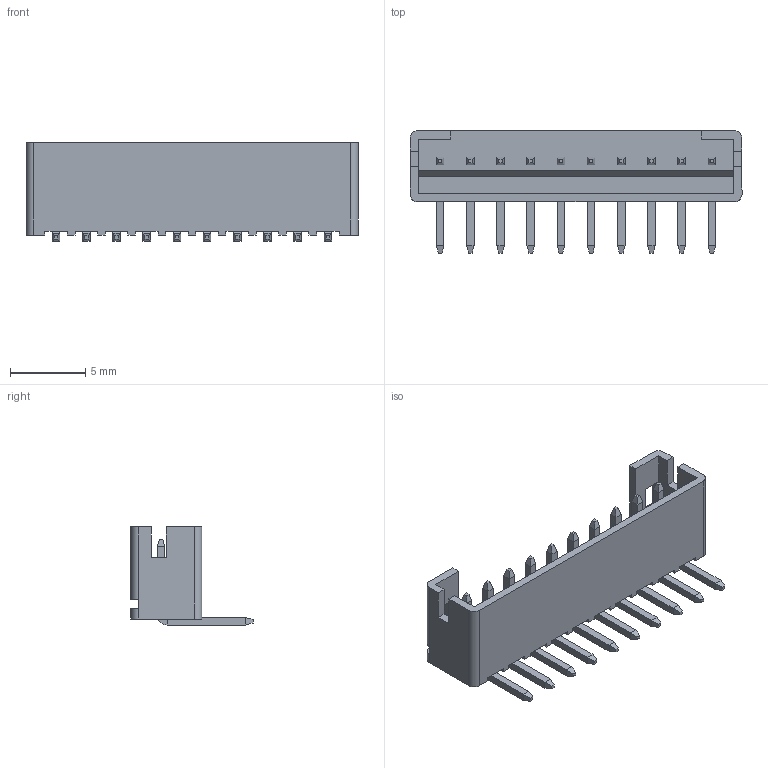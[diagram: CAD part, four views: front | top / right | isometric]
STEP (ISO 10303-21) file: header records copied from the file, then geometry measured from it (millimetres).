
FILE_DESCRIPTION (( 'STEP AP203' ), '1' );
FILE_NAME ('140-510-415-100.STEP', '2020-09-25T11:00:47', ( '' ), ( '' ), 'SwSTEP 2.0', 'SolidWorks 2020', '' );
FILE_SCHEMA (( 'CONFIG_CONTROL_DESIGN' ));
Length unit declared in the file: millimetre
Products named in the file (3): 140-510-415-100; RA LI Contact_Str; RA LI Housing_510
Assembly tree (11 placements, depth 2):
  140-510-415-100
    RA LI Housing_510
    RA LI Contact_Str  x10
Bounding box: 22 x 8.1 x 6.5 mm (x, y, z)
Volume: 239.1 mm3; surface area: 903.3 mm2
Topology: 11 solids, 11 shells, 340 faces, 796 edges, 476 vertices
Faces by surface type: plane 314, cylinder 26
Entity records: 5121 total; most frequent: CARTESIAN_POINT 816, ORIENTED_EDGE 800, DIRECTION 728, EDGE_CURVE 400, LINE 384, VECTOR 384, VERTEX_POINT 260, AXIS2_PLACEMENT_3D 172
